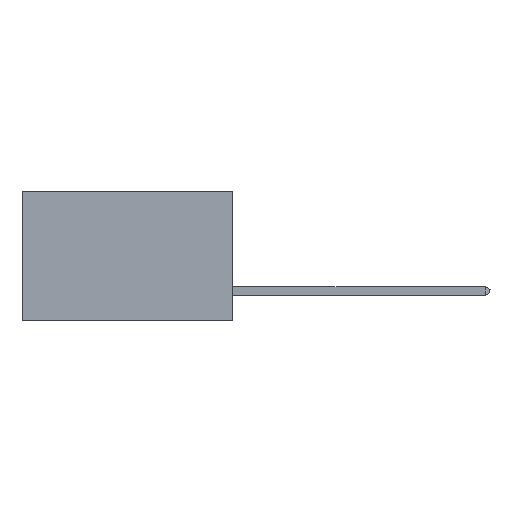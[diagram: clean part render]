
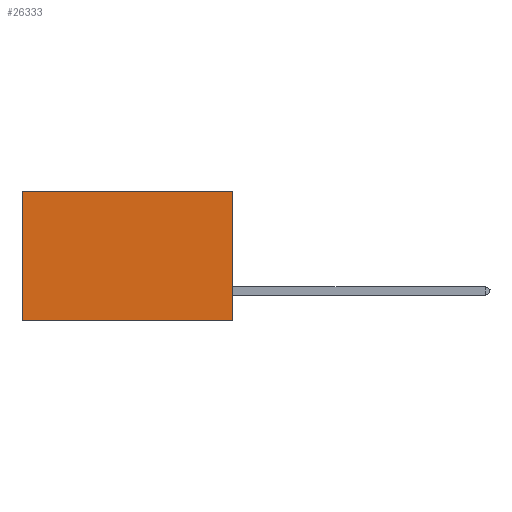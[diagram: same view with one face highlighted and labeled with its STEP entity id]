
A CAD part, left-side view. The second image highlights one B-rep face of the part: STEP entity #26333.
In plain terms, the highlighted planar face has unit normal (-1, 0, 0).
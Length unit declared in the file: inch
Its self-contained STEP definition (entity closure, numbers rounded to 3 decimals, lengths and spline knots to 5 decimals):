
#3948 = CARTESIAN_POINT ( 'NONE',  ( 0.2875, 0.6, -0.37 ) ) ;
#4426 = DIRECTION ( 'NONE',  ( 0., 1., 0. ) ) ;
#6079 = DIRECTION ( 'NONE',  ( 1., 0., 0. ) ) ;
#7872 = CARTESIAN_POINT ( 'NONE',  ( 0.2875, 0., -0.37 ) ) ;
#8040 = CARTESIAN_POINT ( 'NONE',  ( 0.2875, 0., 0. ) ) ;
#8351 = DIRECTION ( 'NONE',  ( 0., 0., -1. ) ) ;
#8820 = VECTOR ( 'NONE', #15095, 39.37008 ) ;
#9399 = CARTESIAN_POINT ( 'NONE',  ( 0.2875, 0., -0.37 ) ) ;
#9756 = ORIENTED_EDGE ( 'NONE', *, *, #18403, .F. ) ;
#10038 = VERTEX_POINT ( 'NONE', #7872 ) ;
#10183 = EDGE_CURVE ( 'NONE', #28673, #20072, #19138, .T. ) ;
#10475 = FACE_OUTER_BOUND ( 'NONE', #18380, .T. ) ;
#13068 = ORIENTED_EDGE ( 'NONE', *, *, #22559, .F. ) ;
#13361 = CARTESIAN_POINT ( 'NONE',  ( 0.2875, 0.6, 0. ) ) ;
#13844 = CARTESIAN_POINT ( 'NONE',  ( 0.2875, 0., 0. ) ) ;
#13963 = DIRECTION ( 'NONE',  ( 0., 0., -1. ) ) ;
#14399 = LINE ( 'NONE', #13844, #29241 ) ;
#15095 = DIRECTION ( 'NONE',  ( 0., 1., 0. ) ) ;
#16105 = LINE ( 'NONE', #18166, #21429 ) ;
#16504 = ORIENTED_EDGE ( 'NONE', *, *, #10183, .T. ) ;
#17234 = AXIS2_PLACEMENT_3D ( 'NONE', #8040, #6079, #8351 ) ;
#17981 = LINE ( 'NONE', #9399, #8820 ) ;
#18166 = CARTESIAN_POINT ( 'NONE',  ( 0.2875, 0.6, 0. ) ) ;
#18380 = EDGE_LOOP ( 'NONE', ( #20266, #13068, #9756, #16504 ) ) ;
#18403 = EDGE_CURVE ( 'NONE', #28673, #10038, #14399, .T. ) ;
#18962 = CARTESIAN_POINT ( 'NONE',  ( 0.2875, 0., 0. ) ) ;
#19040 = EDGE_CURVE ( 'NONE', #20072, #22601, #16105, .T. ) ;
#19138 = LINE ( 'NONE', #20449, #22365 ) ;
#20072 = VERTEX_POINT ( 'NONE', #13361 ) ;
#20266 = ORIENTED_EDGE ( 'NONE', *, *, #19040, .T. ) ;
#20449 = CARTESIAN_POINT ( 'NONE',  ( 0.2875, 0., 0. ) ) ;
#21429 = VECTOR ( 'NONE', #13963, 39.37008 ) ;
#21617 = PLANE ( 'NONE',  #17234 ) ;
#22365 = VECTOR ( 'NONE', #4426, 39.37008 ) ;
#22559 = EDGE_CURVE ( 'NONE', #10038, #22601, #17981, .T. ) ;
#22601 = VERTEX_POINT ( 'NONE', #3948 ) ;
#25083 = DIRECTION ( 'NONE',  ( 0., 0., -1. ) ) ;
#26333 = ADVANCED_FACE ( 'NONE', ( #10475 ), #21617, .F. ) ;
#28673 = VERTEX_POINT ( 'NONE', #18962 ) ;
#29241 = VECTOR ( 'NONE', #25083, 39.37008 ) ;
